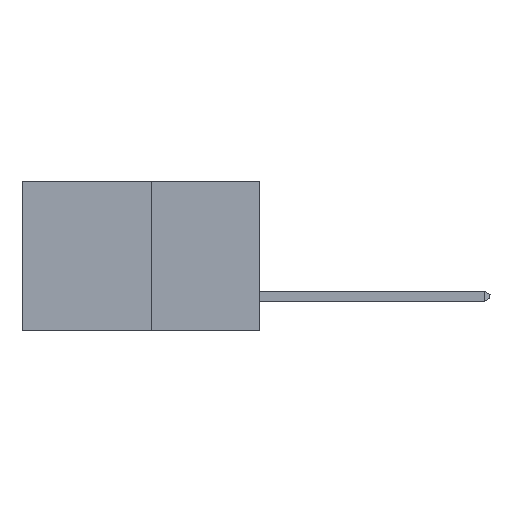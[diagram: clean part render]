
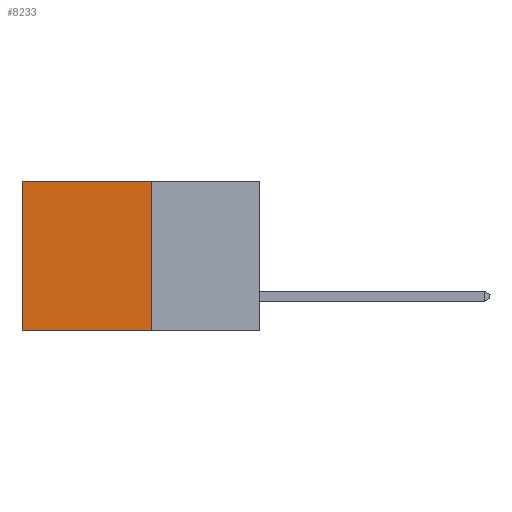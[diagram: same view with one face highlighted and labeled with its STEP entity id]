
A CAD part, left-side view. The second image highlights one B-rep face of the part: STEP entity #8233.
In plain terms, the highlighted planar face has unit normal (-1, 0, 0).
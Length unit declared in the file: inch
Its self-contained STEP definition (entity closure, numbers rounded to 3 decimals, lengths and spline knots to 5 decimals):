
#327 = LINE ( 'NONE', #2972, #5477 ) ;
#613 = CARTESIAN_POINT ( 'NONE',  ( 0.277, 0.59, 0. ) ) ;
#806 = LINE ( 'NONE', #3364, #8569 ) ;
#1247 = CARTESIAN_POINT ( 'NONE',  ( 0.277, 0.27, 0. ) ) ;
#1839 = DIRECTION ( 'NONE',  ( 0., 0., -1. ) ) ;
#1972 = PLANE ( 'NONE',  #2719 ) ;
#2483 = EDGE_CURVE ( 'NONE', #5004, #11303, #10973, .T. ) ;
#2719 = AXIS2_PLACEMENT_3D ( 'NONE', #8075, #9067, #3037 ) ;
#2972 = CARTESIAN_POINT ( 'NONE',  ( 0.277, 0.27, -0.37 ) ) ;
#3037 = DIRECTION ( 'NONE',  ( 0., 0., -1. ) ) ;
#3262 = VECTOR ( 'NONE', #7011, 39.37008 ) ;
#3364 = CARTESIAN_POINT ( 'NONE',  ( 0.277, 0.27, -0.37 ) ) ;
#4436 = DIRECTION ( 'NONE',  ( 0., 1., 0. ) ) ;
#4698 = FACE_OUTER_BOUND ( 'NONE', #11515, .T. ) ;
#5004 = VERTEX_POINT ( 'NONE', #1247 ) ;
#5477 = VECTOR ( 'NONE', #7046, 39.37008 ) ;
#5665 = EDGE_CURVE ( 'NONE', #11303, #7846, #9664, .T. ) ;
#5921 = CARTESIAN_POINT ( 'NONE',  ( 0.277, 0.27, -0.37 ) ) ;
#6234 = EDGE_CURVE ( 'NONE', #5004, #10055, #327, .T. ) ;
#6934 = CARTESIAN_POINT ( 'NONE',  ( 0.277, 0.59, -0.37 ) ) ;
#7011 = DIRECTION ( 'NONE',  ( 0., 1., 0. ) ) ;
#7022 = CARTESIAN_POINT ( 'NONE',  ( 0.277, 0.27, 0. ) ) ;
#7046 = DIRECTION ( 'NONE',  ( 0., 0., -1. ) ) ;
#7732 = ORIENTED_EDGE ( 'NONE', *, *, #8962, .F. ) ;
#7846 = VERTEX_POINT ( 'NONE', #9084 ) ;
#8075 = CARTESIAN_POINT ( 'NONE',  ( 0.277, 0.27, -0.37 ) ) ;
#8233 = ADVANCED_FACE ( 'NONE', ( #4698 ), #1972, .F. ) ;
#8457 = ORIENTED_EDGE ( 'NONE', *, *, #6234, .F. ) ;
#8569 = VECTOR ( 'NONE', #4436, 39.37008 ) ;
#8962 = EDGE_CURVE ( 'NONE', #10055, #7846, #806, .T. ) ;
#9021 = ORIENTED_EDGE ( 'NONE', *, *, #2483, .T. ) ;
#9067 = DIRECTION ( 'NONE',  ( 1., 0., 0. ) ) ;
#9084 = CARTESIAN_POINT ( 'NONE',  ( 0.277, 0.59, -0.37 ) ) ;
#9664 = LINE ( 'NONE', #6934, #12061 ) ;
#10039 = ORIENTED_EDGE ( 'NONE', *, *, #5665, .T. ) ;
#10055 = VERTEX_POINT ( 'NONE', #5921 ) ;
#10973 = LINE ( 'NONE', #7022, #3262 ) ;
#11303 = VERTEX_POINT ( 'NONE', #613 ) ;
#11515 = EDGE_LOOP ( 'NONE', ( #10039, #7732, #8457, #9021 ) ) ;
#12061 = VECTOR ( 'NONE', #1839, 39.37008 ) ;
